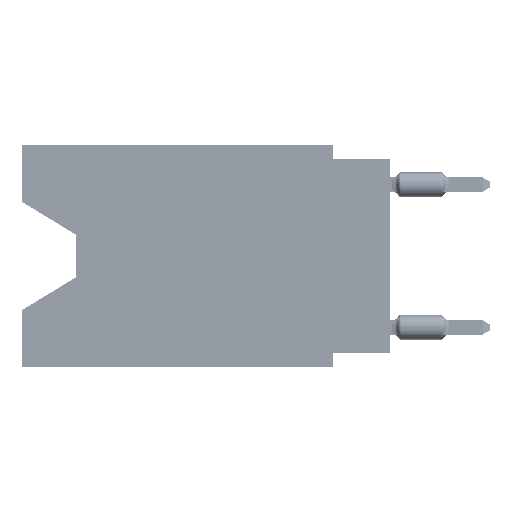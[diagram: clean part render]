
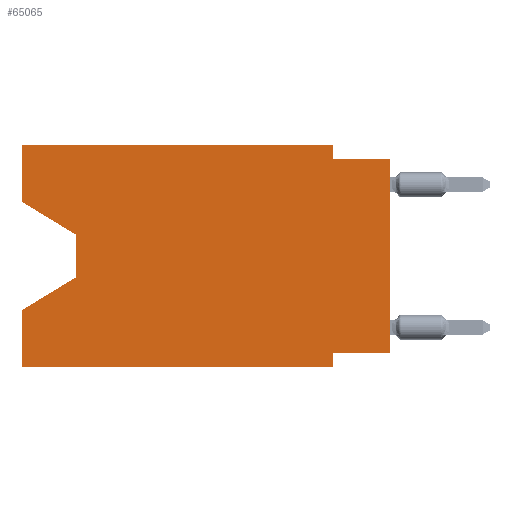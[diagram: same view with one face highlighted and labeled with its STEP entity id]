
A CAD part, left-side view. The second image highlights one B-rep face of the part: STEP entity #65065.
In plain terms, the highlighted planar face has unit normal (-1, 0, 0).
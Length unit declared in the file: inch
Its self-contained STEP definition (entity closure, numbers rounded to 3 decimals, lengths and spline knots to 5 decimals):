
#134 = EDGE_CURVE ( 'NONE', #62713, #57188, #64936, .T. ) ;
#224 = LINE ( 'NONE', #6040, #36876 ) ;
#297 = EDGE_CURVE ( 'NONE', #10211, #4971, #29176, .T. ) ;
#1788 = VECTOR ( 'NONE', #21281, 39.37008 ) ;
#1947 = FACE_OUTER_BOUND ( 'NONE', #10317, .T. ) ;
#2638 = CARTESIAN_POINT ( 'NONE',  ( 0., 0.645, 0. ) ) ;
#3151 = CARTESIAN_POINT ( 'NONE',  ( 0., 0., -0.025 ) ) ;
#3765 = VERTEX_POINT ( 'NONE', #69139 ) ;
#4971 = VERTEX_POINT ( 'NONE', #3151 ) ;
#6040 = CARTESIAN_POINT ( 'NONE',  ( 0., 0.55, -0.232 ) ) ;
#6090 = ORIENTED_EDGE ( 'NONE', *, *, #134, .T. ) ;
#6318 = CARTESIAN_POINT ( 'NONE',  ( 0., 0.1, 0. ) ) ;
#6637 = EDGE_CURVE ( 'NONE', #37278, #68654, #22664, .T. ) ;
#6918 = CARTESIAN_POINT ( 'NONE',  ( 0., 0., -0.025 ) ) ;
#6976 = CARTESIAN_POINT ( 'NONE',  ( 0., 0.645, -0.10025 ) ) ;
#8158 = ORIENTED_EDGE ( 'NONE', *, *, #297, .F. ) ;
#9259 = LINE ( 'NONE', #19839, #14325 ) ;
#9784 = CARTESIAN_POINT ( 'NONE',  ( 0., 0.55, -0.158 ) ) ;
#10150 = AXIS2_PLACEMENT_3D ( 'NONE', #68662, #18700, #40962 ) ;
#10211 = VERTEX_POINT ( 'NONE', #21347 ) ;
#10317 = EDGE_LOOP ( 'NONE', ( #58632, #6090, #34792, #29823, #50803, #32408, #69412, #56452, #8158, #46075, #66548, #65605 ) ) ;
#11130 = CARTESIAN_POINT ( 'NONE',  ( 0., 0., 0. ) ) ;
#11772 = VECTOR ( 'NONE', #49809, 39.37008 ) ;
#11850 = VECTOR ( 'NONE', #57097, 39.37008 ) ;
#12904 = EDGE_CURVE ( 'NONE', #3765, #64950, #9259, .T. ) ;
#13354 = CARTESIAN_POINT ( 'NONE',  ( 0., 0., -0.365 ) ) ;
#14138 = DIRECTION ( 'NONE',  ( 0., 1., 0. ) ) ;
#14325 = VECTOR ( 'NONE', #31141, 39.37008 ) ;
#14672 = VECTOR ( 'NONE', #33970, 39.37008 ) ;
#14976 = DIRECTION ( 'NONE',  ( 0., 0., -1. ) ) ;
#16001 = CARTESIAN_POINT ( 'NONE',  ( 0., 0.645, -0.39 ) ) ;
#16477 = VECTOR ( 'NONE', #14138, 39.37008 ) ;
#16881 = CARTESIAN_POINT ( 'NONE',  ( 0., 0.645, -0.39 ) ) ;
#17276 = VERTEX_POINT ( 'NONE', #6976 ) ;
#18700 = DIRECTION ( 'NONE',  ( 1., 0., 0. ) ) ;
#19482 = LINE ( 'NONE', #35550, #11850 ) ;
#19839 = CARTESIAN_POINT ( 'NONE',  ( 0., 0.645, 0. ) ) ;
#20077 = VECTOR ( 'NONE', #35115, 39.37008 ) ;
#21128 = CARTESIAN_POINT ( 'NONE',  ( 0., 0.1, -0.365 ) ) ;
#21281 = DIRECTION ( 'NONE',  ( 0., 0., -1. ) ) ;
#21347 = CARTESIAN_POINT ( 'NONE',  ( 0., 0.1, -0.025 ) ) ;
#22664 = LINE ( 'NONE', #40536, #14672 ) ;
#23340 = DIRECTION ( 'NONE',  ( 0., -1., 0. ) ) ;
#24185 = PLANE ( 'NONE',  #10150 ) ;
#25887 = DIRECTION ( 'NONE',  ( 0., -1., 0. ) ) ;
#28000 = VECTOR ( 'NONE', #14976, 39.37008 ) ;
#29176 = LINE ( 'NONE', #6918, #39698 ) ;
#29289 = LINE ( 'NONE', #2638, #20077 ) ;
#29823 = ORIENTED_EDGE ( 'NONE', *, *, #6637, .F. ) ;
#30296 = VERTEX_POINT ( 'NONE', #13354 ) ;
#31141 = DIRECTION ( 'NONE',  ( 0., -1., 0. ) ) ;
#31585 = LINE ( 'NONE', #69872, #65675 ) ;
#32408 = ORIENTED_EDGE ( 'NONE', *, *, #39987, .F. ) ;
#33000 = EDGE_CURVE ( 'NONE', #30296, #4971, #39215, .T. ) ;
#33970 = DIRECTION ( 'NONE',  ( 0., 0., 1. ) ) ;
#34792 = ORIENTED_EDGE ( 'NONE', *, *, #64485, .T. ) ;
#35115 = DIRECTION ( 'NONE',  ( 0., 0., 1. ) ) ;
#35315 = EDGE_CURVE ( 'NONE', #37278, #50036, #65609, .T. ) ;
#35550 = CARTESIAN_POINT ( 'NONE',  ( 0., 0.645, -0.10025 ) ) ;
#36876 = VECTOR ( 'NONE', #67293, 39.37008 ) ;
#37278 = VERTEX_POINT ( 'NONE', #16881 ) ;
#39215 = LINE ( 'NONE', #11130, #11772 ) ;
#39698 = VECTOR ( 'NONE', #23340, 39.37008 ) ;
#39987 = EDGE_CURVE ( 'NONE', #67381, #50036, #71213, .T. ) ;
#40536 = CARTESIAN_POINT ( 'NONE',  ( 0., 0.645, 0. ) ) ;
#40962 = DIRECTION ( 'NONE',  ( 0., 0., -1. ) ) ;
#42001 = CARTESIAN_POINT ( 'NONE',  ( 0., 0.55, -0.158 ) ) ;
#45834 = VECTOR ( 'NONE', #25887, 39.37008 ) ;
#46075 = ORIENTED_EDGE ( 'NONE', *, *, #69410, .F. ) ;
#49809 = DIRECTION ( 'NONE',  ( 0., 0., 1. ) ) ;
#50036 = VERTEX_POINT ( 'NONE', #59934 ) ;
#50803 = ORIENTED_EDGE ( 'NONE', *, *, #35315, .T. ) ;
#51279 = EDGE_CURVE ( 'NONE', #17276, #62713, #19482, .T. ) ;
#51690 = EDGE_CURVE ( 'NONE', #17276, #3765, #29289, .T. ) ;
#54188 = DIRECTION ( 'NONE',  ( 0., 0., -1. ) ) ;
#54641 = EDGE_CURVE ( 'NONE', #30296, #67381, #58290, .T. ) ;
#54835 = CARTESIAN_POINT ( 'NONE',  ( 0., 0.1, -0.39 ) ) ;
#56452 = ORIENTED_EDGE ( 'NONE', *, *, #33000, .T. ) ;
#57097 = DIRECTION ( 'NONE',  ( 0., -0.855, -0.519 ) ) ;
#57188 = VERTEX_POINT ( 'NONE', #64922 ) ;
#58290 = LINE ( 'NONE', #58999, #16477 ) ;
#58632 = ORIENTED_EDGE ( 'NONE', *, *, #51279, .T. ) ;
#58999 = CARTESIAN_POINT ( 'NONE',  ( 0., 0., -0.365 ) ) ;
#59934 = CARTESIAN_POINT ( 'NONE',  ( 0., 0.1, -0.39 ) ) ;
#62713 = VERTEX_POINT ( 'NONE', #9784 ) ;
#64485 = EDGE_CURVE ( 'NONE', #57188, #68654, #224, .T. ) ;
#64922 = CARTESIAN_POINT ( 'NONE',  ( 0., 0.55, -0.232 ) ) ;
#64936 = LINE ( 'NONE', #42001, #28000 ) ;
#64950 = VERTEX_POINT ( 'NONE', #6318 ) ;
#65065 = ADVANCED_FACE ( 'NONE', ( #1947 ), #24185, .F. ) ;
#65357 = CARTESIAN_POINT ( 'NONE',  ( 0., 0.645, -0.28975 ) ) ;
#65605 = ORIENTED_EDGE ( 'NONE', *, *, #51690, .F. ) ;
#65609 = LINE ( 'NONE', #16001, #45834 ) ;
#65675 = VECTOR ( 'NONE', #54188, 39.37008 ) ;
#66548 = ORIENTED_EDGE ( 'NONE', *, *, #12904, .F. ) ;
#67293 = DIRECTION ( 'NONE',  ( 0., 0.855, -0.519 ) ) ;
#67381 = VERTEX_POINT ( 'NONE', #21128 ) ;
#68654 = VERTEX_POINT ( 'NONE', #65357 ) ;
#68662 = CARTESIAN_POINT ( 'NONE',  ( 0., 0.645, 0. ) ) ;
#69139 = CARTESIAN_POINT ( 'NONE',  ( 0., 0.645, 0. ) ) ;
#69410 = EDGE_CURVE ( 'NONE', #64950, #10211, #31585, .T. ) ;
#69412 = ORIENTED_EDGE ( 'NONE', *, *, #54641, .F. ) ;
#69872 = CARTESIAN_POINT ( 'NONE',  ( 0., 0.1, 0. ) ) ;
#71213 = LINE ( 'NONE', #54835, #1788 ) ;
